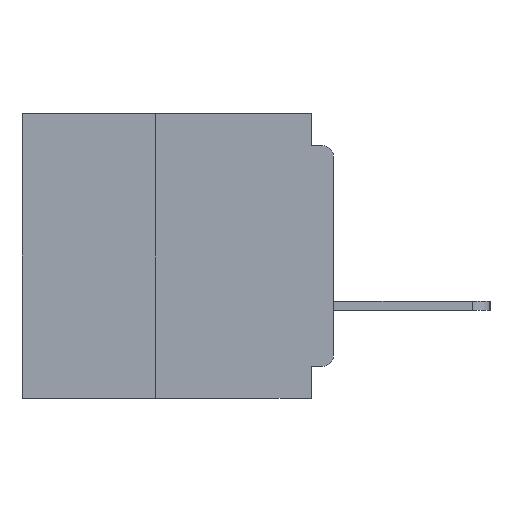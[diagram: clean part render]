
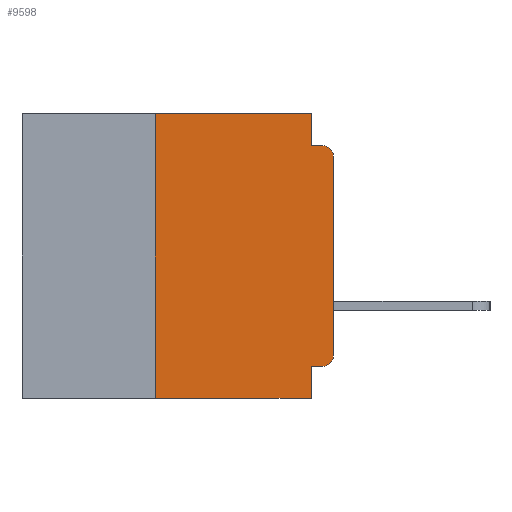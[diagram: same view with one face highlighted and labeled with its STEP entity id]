
A CAD part, left-side view. The second image highlights one B-rep face of the part: STEP entity #9598.
In plain terms, the highlighted planar face has unit normal (-1, 0, 0).
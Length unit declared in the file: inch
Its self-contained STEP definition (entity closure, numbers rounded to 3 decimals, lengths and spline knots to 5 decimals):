
#90 = PLANE ( 'NONE',  #19247 ) ;
#736 = DIRECTION ( 'NONE',  ( 0., 0., -1. ) ) ;
#1730 = VERTEX_POINT ( 'NONE', #2369 ) ;
#2248 = ORIENTED_EDGE ( 'NONE', *, *, #7834, .T. ) ;
#2369 = CARTESIAN_POINT ( 'NONE',  ( 0., 0., -0.34 ) ) ;
#2689 = EDGE_CURVE ( 'NONE', #4003, #32496, #14785, .T. ) ;
#3172 = LINE ( 'NONE', #5938, #9678 ) ;
#3760 = VERTEX_POINT ( 'NONE', #17685 ) ;
#3842 = CARTESIAN_POINT ( 'NONE',  ( 0., 0.015, -0.06 ) ) ;
#3994 = LINE ( 'NONE', #26480, #31891 ) ;
#4003 = VERTEX_POINT ( 'NONE', #7562 ) ;
#4239 = DIRECTION ( 'NONE',  ( -1., 0., 0. ) ) ;
#4490 = VERTEX_POINT ( 'NONE', #15187 ) ;
#5305 = CARTESIAN_POINT ( 'NONE',  ( 0., 0.031, 0. ) ) ;
#5601 = ORIENTED_EDGE ( 'NONE', *, *, #28640, .F. ) ;
#5636 = LINE ( 'NONE', #22011, #27043 ) ;
#5746 = EDGE_LOOP ( 'NONE', ( #14907, #31586, #24743, #26006, #24088, #13571, #26051, #19904, #5601, #2248 ) ) ;
#5938 = CARTESIAN_POINT ( 'NONE',  ( 0., 0.437, 0. ) ) ;
#6324 = CARTESIAN_POINT ( 'NONE',  ( 0., 0., -0.045 ) ) ;
#6429 = VERTEX_POINT ( 'NONE', #8747 ) ;
#6660 = DIRECTION ( 'NONE',  ( 0., 0., -1. ) ) ;
#7403 = VECTOR ( 'NONE', #13272, 39.37008 ) ;
#7562 = CARTESIAN_POINT ( 'NONE',  ( 0., 0.25, -0.4 ) ) ;
#7834 = EDGE_CURVE ( 'NONE', #6429, #1730, #20229, .T. ) ;
#8542 = CARTESIAN_POINT ( 'NONE',  ( 0., 0.437, 0. ) ) ;
#8747 = CARTESIAN_POINT ( 'NONE',  ( 0., 0.015, -0.355 ) ) ;
#9562 = LINE ( 'NONE', #6324, #22710 ) ;
#9598 = ADVANCED_FACE ( 'NONE', ( #34544 ), #90, .F. ) ;
#9678 = VECTOR ( 'NONE', #31036, 39.37008 ) ;
#11186 = LINE ( 'NONE', #34082, #25220 ) ;
#12410 = EDGE_CURVE ( 'NONE', #1730, #3760, #24050, .T. ) ;
#12611 = EDGE_CURVE ( 'NONE', #22436, #21017, #9562, .T. ) ;
#13272 = DIRECTION ( 'NONE',  ( 0., 0., 1. ) ) ;
#13310 = CARTESIAN_POINT ( 'NONE',  ( 0., 0.25, -0.4 ) ) ;
#13550 = VERTEX_POINT ( 'NONE', #16258 ) ;
#13571 = ORIENTED_EDGE ( 'NONE', *, *, #2689, .F. ) ;
#13615 = CIRCLE ( 'NONE', #28087, 0.015 ) ;
#13698 = CARTESIAN_POINT ( 'NONE',  ( 0., 0.25, 0. ) ) ;
#14123 = DIRECTION ( 'NONE',  ( 1., 0., 0. ) ) ;
#14785 = LINE ( 'NONE', #13310, #7403 ) ;
#14907 = ORIENTED_EDGE ( 'NONE', *, *, #12410, .T. ) ;
#15187 = CARTESIAN_POINT ( 'NONE',  ( 0., 0.031, -0.4 ) ) ;
#16258 = CARTESIAN_POINT ( 'NONE',  ( 0., 0.031, 0. ) ) ;
#17685 = CARTESIAN_POINT ( 'NONE',  ( 0., 0., -0.06 ) ) ;
#17905 = CARTESIAN_POINT ( 'NONE',  ( 0., 0.031, -0.045 ) ) ;
#18138 = DIRECTION ( 'NONE',  ( 0., -1., 0. ) ) ;
#19247 = AXIS2_PLACEMENT_3D ( 'NONE', #8542, #14123, #33573 ) ;
#19357 = DIRECTION ( 'NONE',  ( 0., 0., -1. ) ) ;
#19904 = ORIENTED_EDGE ( 'NONE', *, *, #25097, .F. ) ;
#20229 = CIRCLE ( 'NONE', #35198, 0.015 ) ;
#20978 = CARTESIAN_POINT ( 'NONE',  ( 0., 0.015, -0.34 ) ) ;
#21017 = VERTEX_POINT ( 'NONE', #25113 ) ;
#21041 = VECTOR ( 'NONE', #19357, 39.37008 ) ;
#22011 = CARTESIAN_POINT ( 'NONE',  ( 0., 0., -0.355 ) ) ;
#22379 = VERTEX_POINT ( 'NONE', #31658 ) ;
#22436 = VERTEX_POINT ( 'NONE', #17905 ) ;
#22467 = EDGE_CURVE ( 'NONE', #4003, #4490, #3994, .T. ) ;
#22710 = VECTOR ( 'NONE', #28623, 39.37008 ) ;
#23403 = DIRECTION ( 'NONE',  ( -1., 0., 0. ) ) ;
#23817 = DIRECTION ( 'NONE',  ( 0., 0., -1. ) ) ;
#24050 = LINE ( 'NONE', #30579, #36066 ) ;
#24088 = ORIENTED_EDGE ( 'NONE', *, *, #27473, .F. ) ;
#24743 = ORIENTED_EDGE ( 'NONE', *, *, #12611, .F. ) ;
#25097 = EDGE_CURVE ( 'NONE', #22379, #4490, #11186, .T. ) ;
#25113 = CARTESIAN_POINT ( 'NONE',  ( 0., 0.015, -0.045 ) ) ;
#25220 = VECTOR ( 'NONE', #736, 39.37008 ) ;
#26006 = ORIENTED_EDGE ( 'NONE', *, *, #32511, .F. ) ;
#26051 = ORIENTED_EDGE ( 'NONE', *, *, #22467, .T. ) ;
#26480 = CARTESIAN_POINT ( 'NONE',  ( 0., 0.437, -0.4 ) ) ;
#27043 = VECTOR ( 'NONE', #33008, 39.37008 ) ;
#27473 = EDGE_CURVE ( 'NONE', #32496, #13550, #3172, .T. ) ;
#27600 = EDGE_CURVE ( 'NONE', #3760, #21017, #13615, .T. ) ;
#28087 = AXIS2_PLACEMENT_3D ( 'NONE', #3842, #23403, #6660 ) ;
#28623 = DIRECTION ( 'NONE',  ( 0., -1., 0. ) ) ;
#28640 = EDGE_CURVE ( 'NONE', #6429, #22379, #5636, .T. ) ;
#29299 = LINE ( 'NONE', #5305, #21041 ) ;
#30579 = CARTESIAN_POINT ( 'NONE',  ( 0., 0., 0. ) ) ;
#31036 = DIRECTION ( 'NONE',  ( 0., -1., 0. ) ) ;
#31586 = ORIENTED_EDGE ( 'NONE', *, *, #27600, .T. ) ;
#31658 = CARTESIAN_POINT ( 'NONE',  ( 0., 0.031, -0.355 ) ) ;
#31891 = VECTOR ( 'NONE', #18138, 39.37008 ) ;
#32496 = VERTEX_POINT ( 'NONE', #13698 ) ;
#32511 = EDGE_CURVE ( 'NONE', #13550, #22436, #29299, .T. ) ;
#33008 = DIRECTION ( 'NONE',  ( 0., 1., 0. ) ) ;
#33333 = DIRECTION ( 'NONE',  ( 0., 0., 1. ) ) ;
#33573 = DIRECTION ( 'NONE',  ( 0., 0., -1. ) ) ;
#34082 = CARTESIAN_POINT ( 'NONE',  ( 0., 0.031, -0.4 ) ) ;
#34544 = FACE_OUTER_BOUND ( 'NONE', #5746, .T. ) ;
#35198 = AXIS2_PLACEMENT_3D ( 'NONE', #20978, #4239, #23817 ) ;
#36066 = VECTOR ( 'NONE', #33333, 39.37008 ) ;
